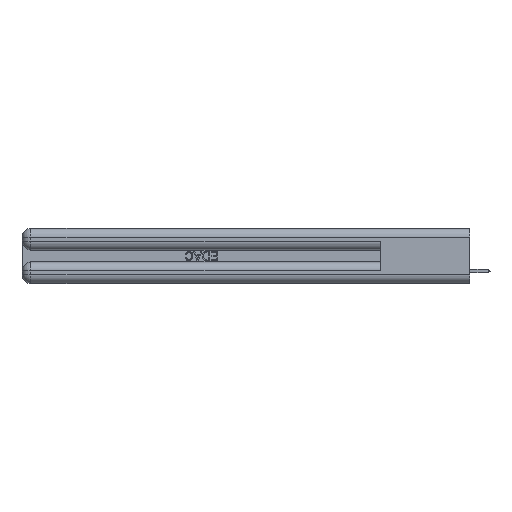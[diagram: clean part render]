
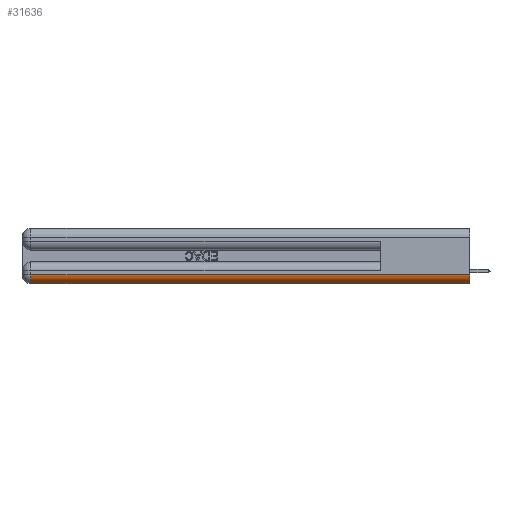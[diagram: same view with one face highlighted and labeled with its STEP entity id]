
A CAD part, left-side view. The second image highlights one B-rep face of the part: STEP entity #31636.
In plain terms, the highlighted cylindrical face has radius 1.524 mm (diameter 3.048 mm), a partial arc.
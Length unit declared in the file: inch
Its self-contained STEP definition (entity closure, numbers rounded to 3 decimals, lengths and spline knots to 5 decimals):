
#1406 = EDGE_CURVE ( 'NONE', #19363, #22489, #3759, .T. ) ;
#1887 = CARTESIAN_POINT ( 'NONE',  ( 0., 0., 0.06 ) ) ;
#2428 = ORIENTED_EDGE ( 'NONE', *, *, #12505, .F. ) ;
#2568 = CARTESIAN_POINT ( 'NONE',  ( 0.06, 0., 0. ) ) ;
#3346 = ORIENTED_EDGE ( 'NONE', *, *, #23156, .F. ) ;
#3759 = LINE ( 'NONE', #29947, #9522 ) ;
#7424 = ORIENTED_EDGE ( 'NONE', *, *, #1406, .F. ) ;
#7639 = DIRECTION ( 'NONE',  ( 0., 0., 1. ) ) ;
#9470 = CARTESIAN_POINT ( 'NONE',  ( 0.06, 0., 0.06 ) ) ;
#9522 = VECTOR ( 'NONE', #26816, 39.37008 ) ;
#9641 = FACE_OUTER_BOUND ( 'NONE', #29112, .T. ) ;
#11371 = VERTEX_POINT ( 'NONE', #28988 ) ;
#11701 = VECTOR ( 'NONE', #34432, 39.37008 ) ;
#11962 = AXIS2_PLACEMENT_3D ( 'NONE', #9470, #35356, #42169 ) ;
#12505 = EDGE_CURVE ( 'NONE', #11371, #19363, #27564, .T. ) ;
#16107 = CYLINDRICAL_SURFACE ( 'NONE', #11962, 0.06 ) ;
#17844 = DIRECTION ( 'NONE',  ( 0., -1., 0. ) ) ;
#19363 = VERTEX_POINT ( 'NONE', #2568 ) ;
#22489 = VERTEX_POINT ( 'NONE', #29983 ) ;
#23156 = EDGE_CURVE ( 'NONE', #39407, #11371, #37747, .T. ) ;
#23823 = CARTESIAN_POINT ( 'NONE',  ( 0.06, 2.94, 0.06 ) ) ;
#26816 = DIRECTION ( 'NONE',  ( 0., 1., 0. ) ) ;
#27107 = DIRECTION ( 'NONE',  ( 0., 1., 0. ) ) ;
#27338 = CARTESIAN_POINT ( 'NONE',  ( 0.06, 0., 0.06 ) ) ;
#27441 = ORIENTED_EDGE ( 'NONE', *, *, #42008, .F. ) ;
#27564 = CIRCLE ( 'NONE', #40168, 0.06 ) ;
#28160 = AXIS2_PLACEMENT_3D ( 'NONE', #23823, #27107, #7639 ) ;
#28988 = CARTESIAN_POINT ( 'NONE',  ( 0., 0., 0.06 ) ) ;
#29112 = EDGE_LOOP ( 'NONE', ( #2428, #3346, #27441, #7424 ) ) ;
#29947 = CARTESIAN_POINT ( 'NONE',  ( 0.06, 3., 0. ) ) ;
#29983 = CARTESIAN_POINT ( 'NONE',  ( 0.06, 2.94, 0. ) ) ;
#30366 = CARTESIAN_POINT ( 'NONE',  ( 0., 2.94, 0.06 ) ) ;
#31636 = ADVANCED_FACE ( 'NONE', ( #9641 ), #16107, .T. ) ;
#32131 = CIRCLE ( 'NONE', #28160, 0.06 ) ;
#34432 = DIRECTION ( 'NONE',  ( 0., -1., 0. ) ) ;
#35356 = DIRECTION ( 'NONE',  ( 0., 1., 0. ) ) ;
#37747 = LINE ( 'NONE', #1887, #11701 ) ;
#39407 = VERTEX_POINT ( 'NONE', #30366 ) ;
#40168 = AXIS2_PLACEMENT_3D ( 'NONE', #27338, #17844, #40712 ) ;
#40712 = DIRECTION ( 'NONE',  ( 0., 0., 1. ) ) ;
#42008 = EDGE_CURVE ( 'NONE', #22489, #39407, #32131, .T. ) ;
#42169 = DIRECTION ( 'NONE',  ( 0., 0., 1. ) ) ;
